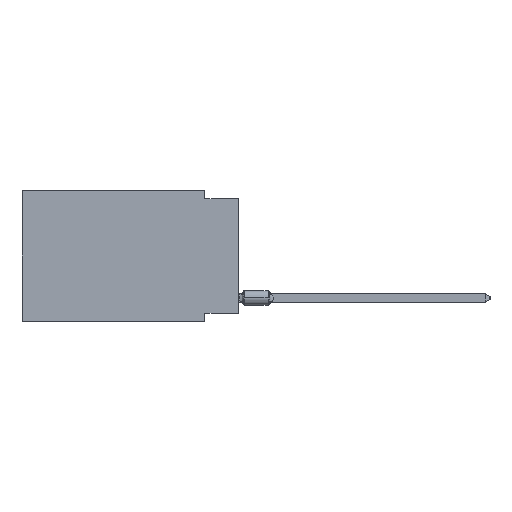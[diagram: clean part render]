
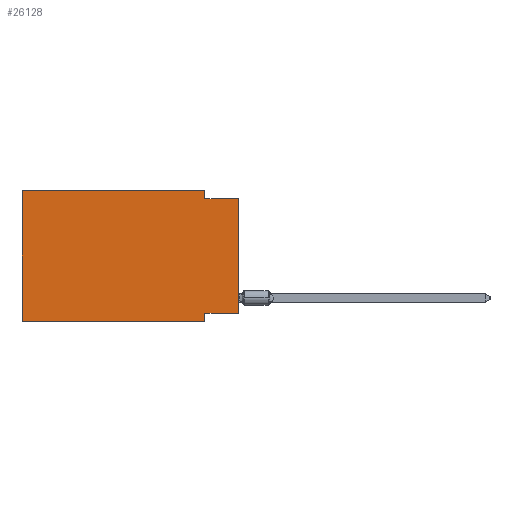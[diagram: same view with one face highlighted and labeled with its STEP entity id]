
A CAD part, left-side view. The second image highlights one B-rep face of the part: STEP entity #26128.
In plain terms, the highlighted planar face has unit normal (-1, 0, 0).
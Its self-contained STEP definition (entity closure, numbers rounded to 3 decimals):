
#905 = CARTESIAN_POINT ( 'NONE',  ( 0., 16.383, 0. ) ) ;
#2356 = VERTEX_POINT ( 'NONE', #17856 ) ;
#2417 = DIRECTION ( 'NONE',  ( 0., 0., -1. ) ) ;
#2918 = EDGE_CURVE ( 'NONE', #19593, #18625, #22183, .T. ) ;
#3413 = DIRECTION ( 'NONE',  ( 1., 0., 0. ) ) ;
#4041 = CARTESIAN_POINT ( 'NONE',  ( 0., 2.54, -9.271 ) ) ;
#4182 = VECTOR ( 'NONE', #43170, 1000. ) ;
#4443 = DIRECTION ( 'NONE',  ( 0., 0., 1. ) ) ;
#4608 = EDGE_CURVE ( 'NONE', #31155, #28971, #29504, .T. ) ;
#5357 = LINE ( 'NONE', #22661, #39593 ) ;
#6681 = EDGE_CURVE ( 'NONE', #38535, #19941, #24393, .T. ) ;
#7287 = ORIENTED_EDGE ( 'NONE', *, *, #17725, .F. ) ;
#7631 = LINE ( 'NONE', #42007, #21020 ) ;
#8329 = ORIENTED_EDGE ( 'NONE', *, *, #42552, .F. ) ;
#9172 = LINE ( 'NONE', #39462, #4182 ) ;
#9435 = CARTESIAN_POINT ( 'NONE',  ( 0., 0., -9.271 ) ) ;
#10303 = ORIENTED_EDGE ( 'NONE', *, *, #4608, .F. ) ;
#10793 = DIRECTION ( 'NONE',  ( 0., -1., 0. ) ) ;
#11223 = AXIS2_PLACEMENT_3D ( 'NONE', #20113, #3413, #34184 ) ;
#12308 = LINE ( 'NONE', #26364, #27038 ) ;
#12530 = EDGE_CURVE ( 'NONE', #19593, #19941, #25955, .T. ) ;
#12807 = ORIENTED_EDGE ( 'NONE', *, *, #35815, .T. ) ;
#14445 = ORIENTED_EDGE ( 'NONE', *, *, #12530, .T. ) ;
#16495 = ORIENTED_EDGE ( 'NONE', *, *, #6681, .F. ) ;
#16640 = ORIENTED_EDGE ( 'NONE', *, *, #2918, .F. ) ;
#16909 = EDGE_LOOP ( 'NONE', ( #14445, #16495, #7287, #10303, #8329, #12807, #30417, #16640 ) ) ;
#17023 = VECTOR ( 'NONE', #35806, 1000. ) ;
#17725 = EDGE_CURVE ( 'NONE', #28971, #38535, #7631, .T. ) ;
#17856 = CARTESIAN_POINT ( 'NONE',  ( 0., 2.54, -9.906 ) ) ;
#18566 = VERTEX_POINT ( 'NONE', #38649 ) ;
#18625 = VERTEX_POINT ( 'NONE', #4041 ) ;
#18952 = CARTESIAN_POINT ( 'NONE',  ( 0., 0., -9.271 ) ) ;
#19593 = VERTEX_POINT ( 'NONE', #18952 ) ;
#19632 = CARTESIAN_POINT ( 'NONE',  ( 0., 16.383, 0. ) ) ;
#19941 = VERTEX_POINT ( 'NONE', #40768 ) ;
#19966 = EDGE_CURVE ( 'NONE', #18625, #2356, #9172, .T. ) ;
#20113 = CARTESIAN_POINT ( 'NONE',  ( 0., 16.383, 0. ) ) ;
#20953 = PLANE ( 'NONE',  #11223 ) ;
#21020 = VECTOR ( 'NONE', #2417, 1000. ) ;
#22134 = DIRECTION ( 'NONE',  ( 0., -1., 0. ) ) ;
#22183 = LINE ( 'NONE', #9435, #17023 ) ;
#22661 = CARTESIAN_POINT ( 'NONE',  ( 0., 16.383, 0. ) ) ;
#24393 = LINE ( 'NONE', #28096, #34837 ) ;
#25671 = DIRECTION ( 'NONE',  ( 0., -1., 0. ) ) ;
#25723 = DIRECTION ( 'NONE',  ( 0., 0., 1. ) ) ;
#25955 = LINE ( 'NONE', #40488, #30889 ) ;
#26128 = ADVANCED_FACE ( 'NONE', ( #45661 ), #20953, .F. ) ;
#26364 = CARTESIAN_POINT ( 'NONE',  ( 0., 16.383, -9.906 ) ) ;
#27038 = VECTOR ( 'NONE', #25671, 1000. ) ;
#28096 = CARTESIAN_POINT ( 'NONE',  ( 0., 0., -0.635 ) ) ;
#28971 = VERTEX_POINT ( 'NONE', #45031 ) ;
#29504 = LINE ( 'NONE', #905, #31850 ) ;
#30417 = ORIENTED_EDGE ( 'NONE', *, *, #19966, .F. ) ;
#30889 = VECTOR ( 'NONE', #25723, 1000. ) ;
#31155 = VERTEX_POINT ( 'NONE', #19632 ) ;
#31850 = VECTOR ( 'NONE', #22134, 1000. ) ;
#34184 = DIRECTION ( 'NONE',  ( 0., 0., -1. ) ) ;
#34837 = VECTOR ( 'NONE', #10793, 1000. ) ;
#35806 = DIRECTION ( 'NONE',  ( 0., 1., 0. ) ) ;
#35815 = EDGE_CURVE ( 'NONE', #18566, #2356, #12308, .T. ) ;
#38535 = VERTEX_POINT ( 'NONE', #40263 ) ;
#38649 = CARTESIAN_POINT ( 'NONE',  ( 0., 16.383, -9.906 ) ) ;
#39462 = CARTESIAN_POINT ( 'NONE',  ( 0., 2.54, -9.906 ) ) ;
#39593 = VECTOR ( 'NONE', #4443, 1000. ) ;
#40263 = CARTESIAN_POINT ( 'NONE',  ( 0., 2.54, -0.635 ) ) ;
#40488 = CARTESIAN_POINT ( 'NONE',  ( 0., 0., 0. ) ) ;
#40768 = CARTESIAN_POINT ( 'NONE',  ( 0., 0., -0.635 ) ) ;
#42007 = CARTESIAN_POINT ( 'NONE',  ( 0., 2.54, 0. ) ) ;
#42552 = EDGE_CURVE ( 'NONE', #18566, #31155, #5357, .T. ) ;
#43170 = DIRECTION ( 'NONE',  ( 0., 0., -1. ) ) ;
#45031 = CARTESIAN_POINT ( 'NONE',  ( 0., 2.54, 0. ) ) ;
#45661 = FACE_OUTER_BOUND ( 'NONE', #16909, .T. ) ;
